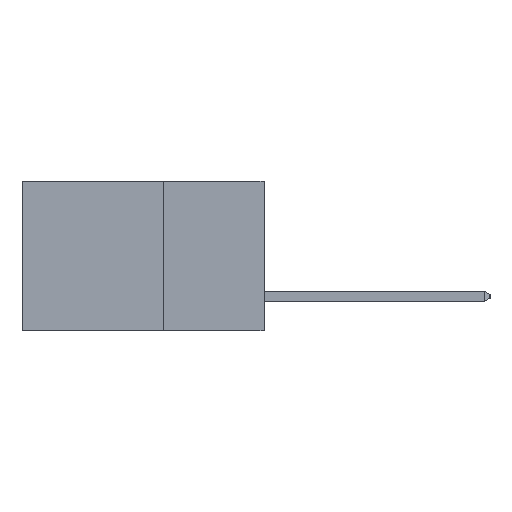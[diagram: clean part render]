
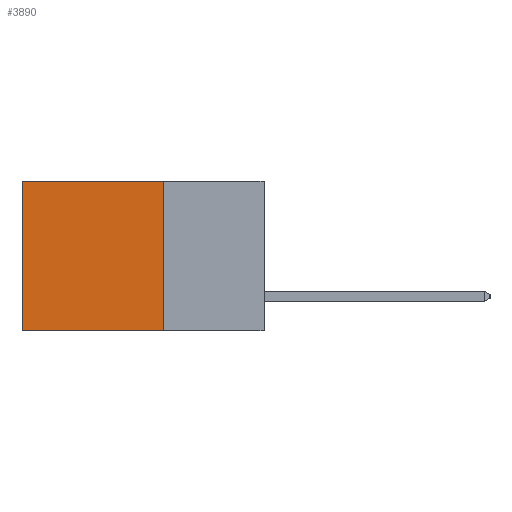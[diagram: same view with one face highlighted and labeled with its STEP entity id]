
A CAD part, left-side view. The second image highlights one B-rep face of the part: STEP entity #3890.
In plain terms, the highlighted planar face has unit normal (-1, 0, 0).
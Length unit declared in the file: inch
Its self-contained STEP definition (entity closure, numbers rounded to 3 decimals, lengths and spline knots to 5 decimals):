
#1402 = ORIENTED_EDGE ( 'NONE', *, *, #9914, .F. ) ;
#1665 = FACE_OUTER_BOUND ( 'NONE', #8688, .T. ) ;
#2635 = LINE ( 'NONE', #7438, #11686 ) ;
#2757 = EDGE_CURVE ( 'NONE', #12364, #4445, #2635, .T. ) ;
#2834 = CARTESIAN_POINT ( 'NONE',  ( 0.2615, 0.25, 0. ) ) ;
#2869 = DIRECTION ( 'NONE',  ( 0., 1., 0. ) ) ;
#3182 = CARTESIAN_POINT ( 'NONE',  ( 0.2615, 0.25, 0. ) ) ;
#3890 = ADVANCED_FACE ( 'NONE', ( #1665 ), #8868, .F. ) ;
#4013 = VECTOR ( 'NONE', #9159, 39.37008 ) ;
#4445 = VERTEX_POINT ( 'NONE', #8549 ) ;
#4687 = VECTOR ( 'NONE', #2869, 39.37008 ) ;
#4735 = CARTESIAN_POINT ( 'NONE',  ( 0.2615, 0.6, -0.37 ) ) ;
#5663 = DIRECTION ( 'NONE',  ( 0., 0., -1. ) ) ;
#5917 = DIRECTION ( 'NONE',  ( 0., 0., -1. ) ) ;
#6931 = VERTEX_POINT ( 'NONE', #7821 ) ;
#7240 = LINE ( 'NONE', #14788, #4013 ) ;
#7438 = CARTESIAN_POINT ( 'NONE',  ( 0.2615, 0.25, -0.37 ) ) ;
#7821 = CARTESIAN_POINT ( 'NONE',  ( 0.2615, 0.6, -0.37 ) ) ;
#8207 = LINE ( 'NONE', #2834, #4687 ) ;
#8527 = EDGE_CURVE ( 'NONE', #12364, #10137, #8207, .T. ) ;
#8549 = CARTESIAN_POINT ( 'NONE',  ( 0.2615, 0.25, -0.37 ) ) ;
#8651 = DIRECTION ( 'NONE',  ( 0., 0., -1. ) ) ;
#8688 = EDGE_LOOP ( 'NONE', ( #14977, #1402, #10404, #13842 ) ) ;
#8804 = DIRECTION ( 'NONE',  ( 1., 0., 0. ) ) ;
#8868 = PLANE ( 'NONE',  #8890 ) ;
#8890 = AXIS2_PLACEMENT_3D ( 'NONE', #9343, #8804, #8651 ) ;
#9159 = DIRECTION ( 'NONE',  ( 0., 1., 0. ) ) ;
#9343 = CARTESIAN_POINT ( 'NONE',  ( 0.2615, 0.25, -0.37 ) ) ;
#9914 = EDGE_CURVE ( 'NONE', #4445, #6931, #7240, .T. ) ;
#10058 = EDGE_CURVE ( 'NONE', #10137, #6931, #11922, .T. ) ;
#10137 = VERTEX_POINT ( 'NONE', #12935 ) ;
#10404 = ORIENTED_EDGE ( 'NONE', *, *, #2757, .F. ) ;
#11686 = VECTOR ( 'NONE', #5663, 39.37008 ) ;
#11922 = LINE ( 'NONE', #4735, #13839 ) ;
#12364 = VERTEX_POINT ( 'NONE', #3182 ) ;
#12935 = CARTESIAN_POINT ( 'NONE',  ( 0.2615, 0.6, 0. ) ) ;
#13839 = VECTOR ( 'NONE', #5917, 39.37008 ) ;
#13842 = ORIENTED_EDGE ( 'NONE', *, *, #8527, .T. ) ;
#14788 = CARTESIAN_POINT ( 'NONE',  ( 0.2615, 0.25, -0.37 ) ) ;
#14977 = ORIENTED_EDGE ( 'NONE', *, *, #10058, .T. ) ;
